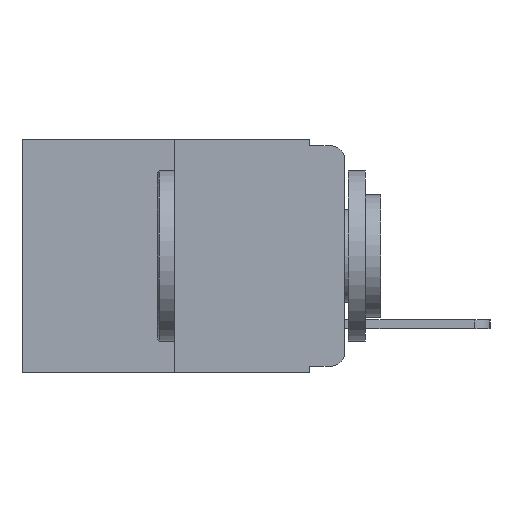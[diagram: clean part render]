
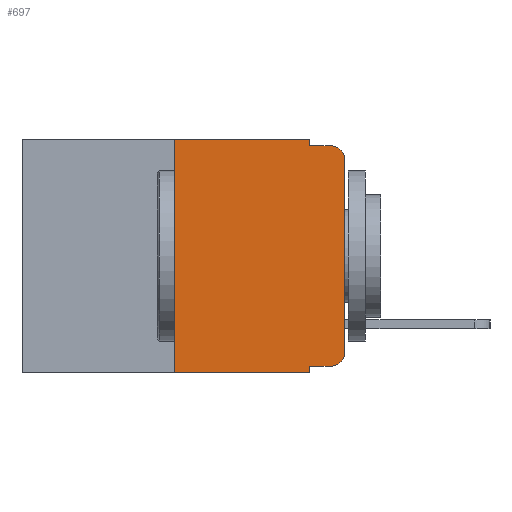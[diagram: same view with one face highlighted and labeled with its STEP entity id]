
A CAD part, left-side view. The second image highlights one B-rep face of the part: STEP entity #697.
In plain terms, the highlighted planar face has unit normal (-1, 0, 0).
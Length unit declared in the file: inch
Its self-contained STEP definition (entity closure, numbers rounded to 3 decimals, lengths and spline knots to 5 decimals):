
#4 = CARTESIAN_POINT ( 'NONE',  ( 0., 0.02, -0.03 ) ) ;
#680 = DIRECTION ( 'NONE',  ( -1., 0., 0. ) ) ;
#697 = ADVANCED_FACE ( 'NONE', ( #21758 ), #18825, .F. ) ;
#1434 = EDGE_CURVE ( 'NONE', #7334, #17011, #2463, .T. ) ;
#2063 = DIRECTION ( 'NONE',  ( 0., 0., -1. ) ) ;
#2175 = EDGE_CURVE ( 'NONE', #7142, #5129, #10657, .T. ) ;
#2463 = LINE ( 'NONE', #10224, #17666 ) ;
#3049 = EDGE_LOOP ( 'NONE', ( #4824, #5297, #5617, #6077, #6274, #6856, #8476, #8541, #8640, #9200 ) ) ;
#3305 = DIRECTION ( 'NONE',  ( 0., -1., 0. ) ) ;
#3309 = EDGE_CURVE ( 'NONE', #5129, #5372, #17943, .T. ) ;
#3395 = VECTOR ( 'NONE', #14720, 39.37008 ) ;
#3726 = CARTESIAN_POINT ( 'NONE',  ( 0., 0.051, -0.343 ) ) ;
#4393 = CARTESIAN_POINT ( 'NONE',  ( 0., 0., -0.313 ) ) ;
#4824 = ORIENTED_EDGE ( 'NONE', *, *, #1434, .T. ) ;
#4891 = VECTOR ( 'NONE', #13738, 39.37008 ) ;
#5129 = VERTEX_POINT ( 'NONE', #21648 ) ;
#5297 = ORIENTED_EDGE ( 'NONE', *, *, #10325, .T. ) ;
#5372 = VERTEX_POINT ( 'NONE', #23588 ) ;
#5615 = DIRECTION ( 'NONE',  ( 0., 0., 1. ) ) ;
#5617 = ORIENTED_EDGE ( 'NONE', *, *, #3309, .F. ) ;
#5822 = DIRECTION ( 'NONE',  ( 0., 0., -1. ) ) ;
#6077 = ORIENTED_EDGE ( 'NONE', *, *, #2175, .F. ) ;
#6274 = ORIENTED_EDGE ( 'NONE', *, *, #19089, .F. ) ;
#6445 = CARTESIAN_POINT ( 'NONE',  ( 0., 0.473, -0.343 ) ) ;
#6822 = CIRCLE ( 'NONE', #23418, 0.02 ) ;
#6856 = ORIENTED_EDGE ( 'NONE', *, *, #21810, .F. ) ;
#7142 = VERTEX_POINT ( 'NONE', #19953 ) ;
#7334 = VERTEX_POINT ( 'NONE', #4393 ) ;
#8455 = CARTESIAN_POINT ( 'NONE',  ( 0., 0., -0.03 ) ) ;
#8476 = ORIENTED_EDGE ( 'NONE', *, *, #22660, .T. ) ;
#8541 = ORIENTED_EDGE ( 'NONE', *, *, #9077, .F. ) ;
#8640 = ORIENTED_EDGE ( 'NONE', *, *, #18530, .T. ) ;
#8887 = AXIS2_PLACEMENT_3D ( 'NONE', #17151, #17912, #16497 ) ;
#9077 = EDGE_CURVE ( 'NONE', #19792, #15346, #20279, .T. ) ;
#9200 = ORIENTED_EDGE ( 'NONE', *, *, #16940, .T. ) ;
#9293 = LINE ( 'NONE', #9349, #22845 ) ;
#9349 = CARTESIAN_POINT ( 'NONE',  ( 0., 0.25, 0. ) ) ;
#10224 = CARTESIAN_POINT ( 'NONE',  ( 0., 0., 0. ) ) ;
#10241 = VERTEX_POINT ( 'NONE', #11267 ) ;
#10325 = EDGE_CURVE ( 'NONE', #17011, #5372, #6822, .T. ) ;
#10515 = DIRECTION ( 'NONE',  ( 0., 0., 1. ) ) ;
#10657 = LINE ( 'NONE', #20107, #23514 ) ;
#11267 = CARTESIAN_POINT ( 'NONE',  ( 0., 0.25, 0. ) ) ;
#11990 = CARTESIAN_POINT ( 'NONE',  ( 0., 0.02, -0.313 ) ) ;
#13183 = DIRECTION ( 'NONE',  ( -1., 0., 0. ) ) ;
#13738 = DIRECTION ( 'NONE',  ( 0., -1., 0. ) ) ;
#13754 = DIRECTION ( 'NONE',  ( 0., 0., -1. ) ) ;
#14147 = VERTEX_POINT ( 'NONE', #19929 ) ;
#14185 = LINE ( 'NONE', #15499, #22938 ) ;
#14203 = LINE ( 'NONE', #17903, #22958 ) ;
#14559 = LINE ( 'NONE', #6445, #4891 ) ;
#14720 = DIRECTION ( 'NONE',  ( 0., -1., 0. ) ) ;
#15346 = VERTEX_POINT ( 'NONE', #3726 ) ;
#15384 = CARTESIAN_POINT ( 'NONE',  ( 0., 0.051, 0. ) ) ;
#15499 = CARTESIAN_POINT ( 'NONE',  ( 0., 0.473, 0. ) ) ;
#16429 = VERTEX_POINT ( 'NONE', #19416 ) ;
#16497 = DIRECTION ( 'NONE',  ( 0., 0., -1. ) ) ;
#16940 = EDGE_CURVE ( 'NONE', #14147, #7334, #19562, .T. ) ;
#17011 = VERTEX_POINT ( 'NONE', #8455 ) ;
#17151 = CARTESIAN_POINT ( 'NONE',  ( 0., 0.473, 0. ) ) ;
#17666 = VECTOR ( 'NONE', #10515, 39.37008 ) ;
#17775 = AXIS2_PLACEMENT_3D ( 'NONE', #11990, #680, #13754 ) ;
#17903 = CARTESIAN_POINT ( 'NONE',  ( 0., 0.051, -0.333 ) ) ;
#17912 = DIRECTION ( 'NONE',  ( 1., 0., 0. ) ) ;
#17943 = LINE ( 'NONE', #23416, #3395 ) ;
#18530 = EDGE_CURVE ( 'NONE', #19792, #14147, #14203, .T. ) ;
#18825 = PLANE ( 'NONE',  #8887 ) ;
#19089 = EDGE_CURVE ( 'NONE', #10241, #7142, #14185, .T. ) ;
#19416 = CARTESIAN_POINT ( 'NONE',  ( 0., 0.25, -0.343 ) ) ;
#19562 = CIRCLE ( 'NONE', #17775, 0.02 ) ;
#19759 = VECTOR ( 'NONE', #22417, 39.37008 ) ;
#19792 = VERTEX_POINT ( 'NONE', #21922 ) ;
#19929 = CARTESIAN_POINT ( 'NONE',  ( 0., 0.02, -0.333 ) ) ;
#19953 = CARTESIAN_POINT ( 'NONE',  ( 0., 0.051, 0. ) ) ;
#20107 = CARTESIAN_POINT ( 'NONE',  ( 0., 0.051, 0. ) ) ;
#20279 = LINE ( 'NONE', #15384, #19759 ) ;
#21648 = CARTESIAN_POINT ( 'NONE',  ( 0., 0.051, -0.01 ) ) ;
#21758 = FACE_OUTER_BOUND ( 'NONE', #3049, .T. ) ;
#21810 = EDGE_CURVE ( 'NONE', #16429, #10241, #9293, .T. ) ;
#21922 = CARTESIAN_POINT ( 'NONE',  ( 0., 0.051, -0.333 ) ) ;
#22369 = DIRECTION ( 'NONE',  ( 0., -1., 0. ) ) ;
#22417 = DIRECTION ( 'NONE',  ( 0., 0., -1. ) ) ;
#22660 = EDGE_CURVE ( 'NONE', #16429, #15346, #14559, .T. ) ;
#22845 = VECTOR ( 'NONE', #5615, 39.37008 ) ;
#22938 = VECTOR ( 'NONE', #22369, 39.37008 ) ;
#22958 = VECTOR ( 'NONE', #3305, 39.37008 ) ;
#23416 = CARTESIAN_POINT ( 'NONE',  ( 0., 0.051, -0.01 ) ) ;
#23418 = AXIS2_PLACEMENT_3D ( 'NONE', #4, #13183, #2063 ) ;
#23514 = VECTOR ( 'NONE', #5822, 39.37008 ) ;
#23588 = CARTESIAN_POINT ( 'NONE',  ( 0., 0.02, -0.01 ) ) ;
